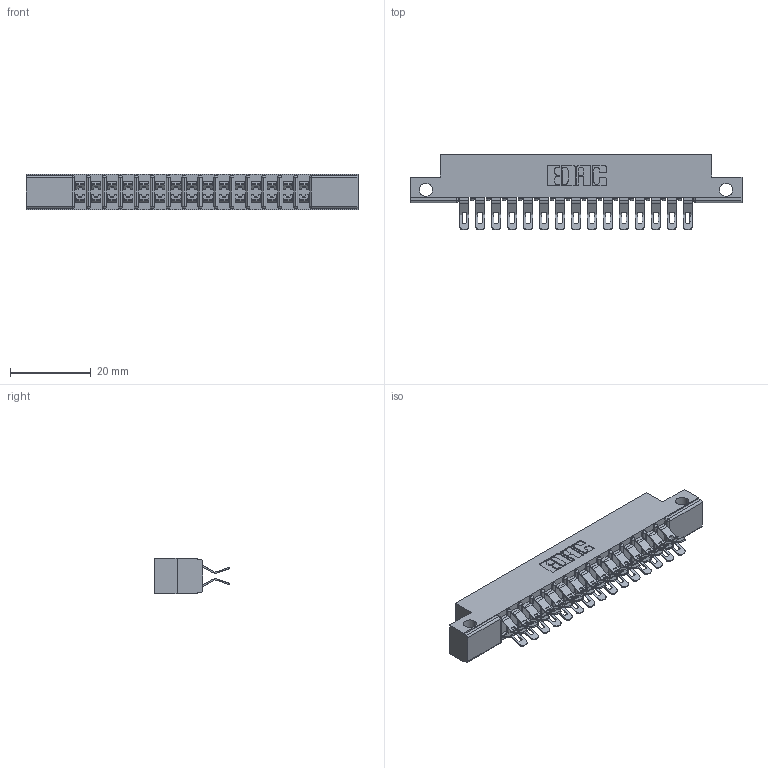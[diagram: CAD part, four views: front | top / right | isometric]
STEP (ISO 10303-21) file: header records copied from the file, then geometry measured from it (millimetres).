
FILE_DESCRIPTION (( 'STEP AP203' ), '1' );
FILE_NAME ('357-030-555-212.STEP', '2019-09-18T00:42:37', ( '' ), ( '' ), 'SwSTEP 2.0', 'SolidWorks 2016', '' );
FILE_SCHEMA (( 'CONFIG_CONTROL_DESIGN' ));
Length unit declared in the file: inch
Products named in the file (3): 307 Part_.128 Dia Side Mounting Holes; 307-290-001_555; 357-030-555-212
Assembly tree (31 placements, depth 2):
  357-030-555-212
    307 Part_.128 Dia Side Mounting Holes
    307-290-001_555  x30
Bounding box: 82.45 x 18.75 x 8.71 mm (x, y, z)
Volume: 5407.3 mm3; surface area: 9540.9 mm2
Topology: 31 solids, 31 shells, 1964 faces, 5753 edges, 3750 vertices
Faces by surface type: plane 1090, cylinder 842, sphere 32
Entity records: 17207 total; most frequent: CARTESIAN_POINT 2827, ORIENTED_EDGE 2800, DIRECTION 2788, EDGE_CURVE 1400, LINE 1050, VECTOR 1050, VERTEX_POINT 908, AXIS2_PLACEMENT_3D 869
